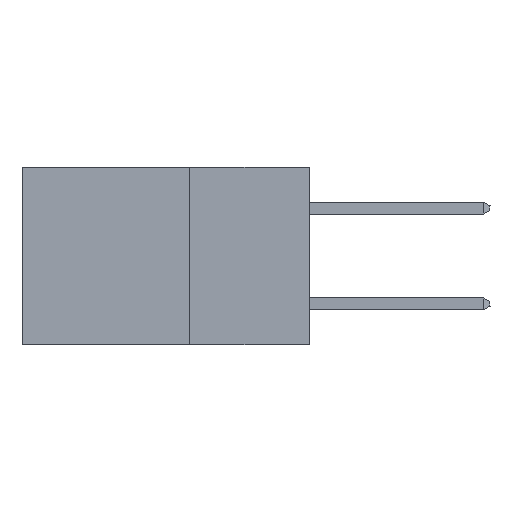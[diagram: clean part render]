
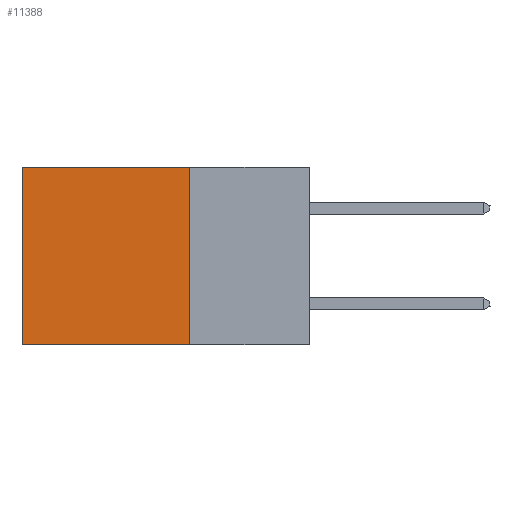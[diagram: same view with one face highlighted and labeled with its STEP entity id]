
A CAD part, left-side view. The second image highlights one B-rep face of the part: STEP entity #11388.
In plain terms, the highlighted planar face has unit normal (-1, 0, 0).
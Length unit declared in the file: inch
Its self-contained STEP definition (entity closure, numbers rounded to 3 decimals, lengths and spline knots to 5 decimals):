
#345 = LINE ( 'NONE', #21624, #4746 ) ;
#637 = ORIENTED_EDGE ( 'NONE', *, *, #10897, .F. ) ;
#876 = VERTEX_POINT ( 'NONE', #19613 ) ;
#1062 = LINE ( 'NONE', #22927, #5473 ) ;
#1365 = CARTESIAN_POINT ( 'NONE',  ( 0.2875, 0.25, 0. ) ) ;
#3154 = ORIENTED_EDGE ( 'NONE', *, *, #4225, .T. ) ;
#3253 = LINE ( 'NONE', #12419, #12580 ) ;
#4225 = EDGE_CURVE ( 'NONE', #7874, #20978, #21919, .T. ) ;
#4436 = ORIENTED_EDGE ( 'NONE', *, *, #19148, .F. ) ;
#4746 = VECTOR ( 'NONE', #18133, 39.37008 ) ;
#5473 = VECTOR ( 'NONE', #8370, 39.37008 ) ;
#5966 = PLANE ( 'NONE',  #19182 ) ;
#6815 = EDGE_LOOP ( 'NONE', ( #3154, #4436, #637, #22464 ) ) ;
#7874 = VERTEX_POINT ( 'NONE', #11880 ) ;
#8370 = DIRECTION ( 'NONE',  ( 0., 0., -1. ) ) ;
#9695 = CARTESIAN_POINT ( 'NONE',  ( 0.2875, 0.25, 0. ) ) ;
#10897 = EDGE_CURVE ( 'NONE', #13997, #876, #1062, .T. ) ;
#11388 = ADVANCED_FACE ( 'NONE', ( #22587 ), #5966, .F. ) ;
#11570 = DIRECTION ( 'NONE',  ( 0., 0., -1. ) ) ;
#11722 = VECTOR ( 'NONE', #16186, 39.37008 ) ;
#11880 = CARTESIAN_POINT ( 'NONE',  ( 0.2875, 0.6, 0. ) ) ;
#12419 = CARTESIAN_POINT ( 'NONE',  ( 0.2875, 0.25, 0. ) ) ;
#12580 = VECTOR ( 'NONE', #14319, 39.37008 ) ;
#13997 = VERTEX_POINT ( 'NONE', #1365 ) ;
#14319 = DIRECTION ( 'NONE',  ( 0., 1., 0. ) ) ;
#14376 = CARTESIAN_POINT ( 'NONE',  ( 0.2875, 0.6, 0. ) ) ;
#15785 = EDGE_CURVE ( 'NONE', #13997, #7874, #3253, .T. ) ;
#16186 = DIRECTION ( 'NONE',  ( 0., 0., -1. ) ) ;
#18133 = DIRECTION ( 'NONE',  ( 0., 1., 0. ) ) ;
#18303 = CARTESIAN_POINT ( 'NONE',  ( 0.2875, 0.6, -0.37 ) ) ;
#19148 = EDGE_CURVE ( 'NONE', #876, #20978, #345, .T. ) ;
#19182 = AXIS2_PLACEMENT_3D ( 'NONE', #9695, #22422, #11570 ) ;
#19613 = CARTESIAN_POINT ( 'NONE',  ( 0.2875, 0.25, -0.37 ) ) ;
#20978 = VERTEX_POINT ( 'NONE', #18303 ) ;
#21624 = CARTESIAN_POINT ( 'NONE',  ( 0.2875, 0.25, -0.37 ) ) ;
#21919 = LINE ( 'NONE', #14376, #11722 ) ;
#22422 = DIRECTION ( 'NONE',  ( 1., 0., 0. ) ) ;
#22464 = ORIENTED_EDGE ( 'NONE', *, *, #15785, .T. ) ;
#22587 = FACE_OUTER_BOUND ( 'NONE', #6815, .T. ) ;
#22927 = CARTESIAN_POINT ( 'NONE',  ( 0.2875, 0.25, 0. ) ) ;
